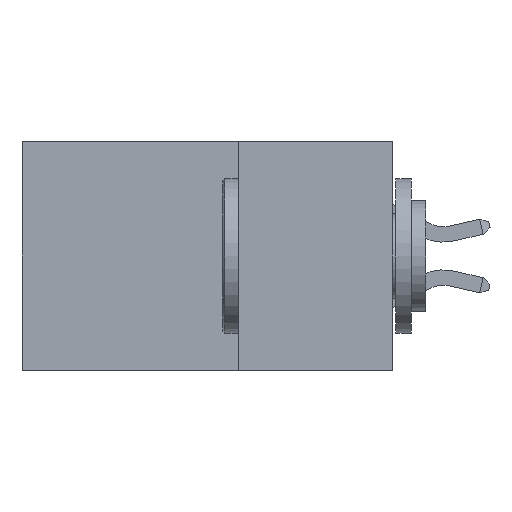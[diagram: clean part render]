
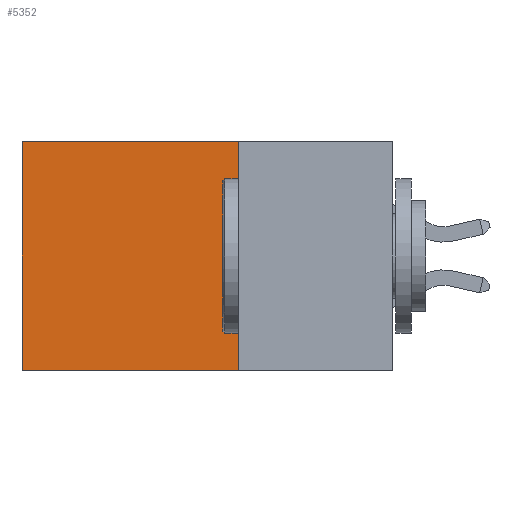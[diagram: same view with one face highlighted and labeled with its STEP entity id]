
A CAD part, left-side view. The second image highlights one B-rep face of the part: STEP entity #5352.
In plain terms, the highlighted planar face has unit normal (-1, 0, 0).
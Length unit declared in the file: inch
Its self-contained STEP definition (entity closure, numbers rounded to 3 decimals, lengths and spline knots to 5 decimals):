
#399 = CARTESIAN_POINT ( 'NONE',  ( 0.2875, 0.6, -0.37 ) ) ;
#744 = VECTOR ( 'NONE', #19595, 39.37008 ) ;
#1423 = EDGE_LOOP ( 'NONE', ( #25001, #11809, #2634, #2837 ) ) ;
#1636 = CARTESIAN_POINT ( 'NONE',  ( 0.2875, 0.25, 0. ) ) ;
#2531 = CARTESIAN_POINT ( 'NONE',  ( 0.2875, 0.6, 0. ) ) ;
#2634 = ORIENTED_EDGE ( 'NONE', *, *, #4707, .F. ) ;
#2837 = ORIENTED_EDGE ( 'NONE', *, *, #24178, .T. ) ;
#3021 = VECTOR ( 'NONE', #8876, 39.37008 ) ;
#4707 = EDGE_CURVE ( 'NONE', #4971, #20926, #18698, .T. ) ;
#4749 = VERTEX_POINT ( 'NONE', #2531 ) ;
#4971 = VERTEX_POINT ( 'NONE', #14681 ) ;
#5352 = ADVANCED_FACE ( 'NONE', ( #10752 ), #21380, .F. ) ;
#6866 = CARTESIAN_POINT ( 'NONE',  ( 0.2875, 0.25, -0.37 ) ) ;
#8235 = AXIS2_PLACEMENT_3D ( 'NONE', #25444, #15097, #15176 ) ;
#8876 = DIRECTION ( 'NONE',  ( 0., 1., 0. ) ) ;
#8961 = LINE ( 'NONE', #6866, #3021 ) ;
#10752 = FACE_OUTER_BOUND ( 'NONE', #1423, .T. ) ;
#11809 = ORIENTED_EDGE ( 'NONE', *, *, #21782, .F. ) ;
#14269 = DIRECTION ( 'NONE',  ( 0., 0., -1. ) ) ;
#14551 = VECTOR ( 'NONE', #14269, 39.37008 ) ;
#14681 = CARTESIAN_POINT ( 'NONE',  ( 0.2875, 0.25, 0. ) ) ;
#15097 = DIRECTION ( 'NONE',  ( 1., 0., 0. ) ) ;
#15176 = DIRECTION ( 'NONE',  ( 0., 0., -1. ) ) ;
#17491 = EDGE_CURVE ( 'NONE', #4749, #22297, #17948, .T. ) ;
#17948 = LINE ( 'NONE', #22984, #23069 ) ;
#18485 = CARTESIAN_POINT ( 'NONE',  ( 0.2875, 0.25, -0.37 ) ) ;
#18698 = LINE ( 'NONE', #20052, #14551 ) ;
#19595 = DIRECTION ( 'NONE',  ( 0., 1., 0. ) ) ;
#20052 = CARTESIAN_POINT ( 'NONE',  ( 0.2875, 0.25, 0. ) ) ;
#20926 = VERTEX_POINT ( 'NONE', #18485 ) ;
#21380 = PLANE ( 'NONE',  #8235 ) ;
#21782 = EDGE_CURVE ( 'NONE', #20926, #22297, #8961, .T. ) ;
#22297 = VERTEX_POINT ( 'NONE', #399 ) ;
#22897 = DIRECTION ( 'NONE',  ( 0., 0., -1. ) ) ;
#22984 = CARTESIAN_POINT ( 'NONE',  ( 0.2875, 0.6, 0. ) ) ;
#23069 = VECTOR ( 'NONE', #22897, 39.37008 ) ;
#23407 = LINE ( 'NONE', #1636, #744 ) ;
#24178 = EDGE_CURVE ( 'NONE', #4971, #4749, #23407, .T. ) ;
#25001 = ORIENTED_EDGE ( 'NONE', *, *, #17491, .T. ) ;
#25444 = CARTESIAN_POINT ( 'NONE',  ( 0.2875, 0.25, 0. ) ) ;
